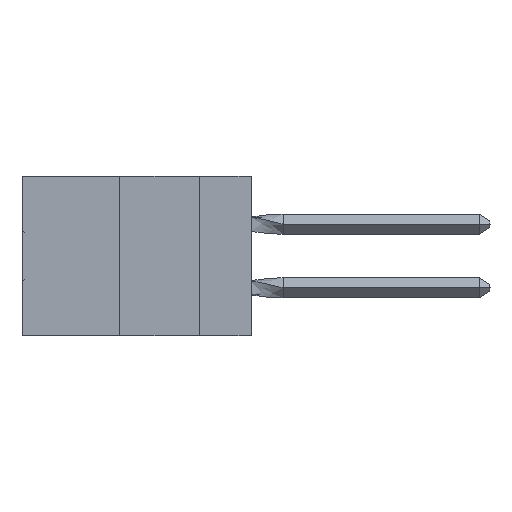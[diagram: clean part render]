
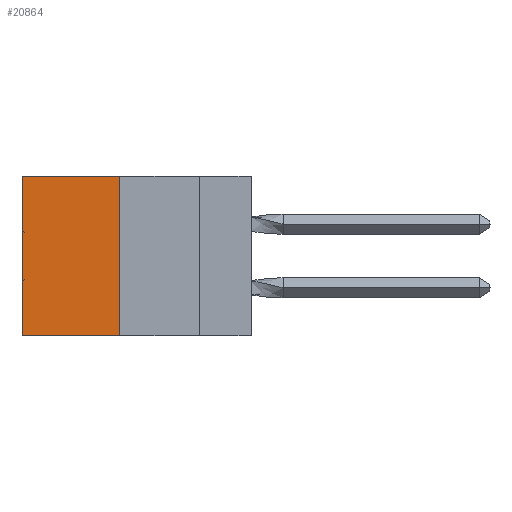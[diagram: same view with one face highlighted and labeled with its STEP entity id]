
A CAD part, left-side view. The second image highlights one B-rep face of the part: STEP entity #20864.
In plain terms, the highlighted planar face has unit normal (-1, 0, 0).
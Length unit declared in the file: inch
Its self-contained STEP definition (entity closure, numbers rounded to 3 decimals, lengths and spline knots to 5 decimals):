
#2740 = EDGE_CURVE ( 'NONE', #23271, #10534, #30842, .T. ) ;
#7665 = VECTOR ( 'NONE', #19204, 39.37008 ) ;
#10534 = VERTEX_POINT ( 'NONE', #34947 ) ;
#11364 = PLANE ( 'NONE',  #20987 ) ;
#13994 = EDGE_CURVE ( 'NONE', #23271, #24695, #32290, .T. ) ;
#16296 = LINE ( 'NONE', #21968, #38997 ) ;
#18318 = ORIENTED_EDGE ( 'NONE', *, *, #45078, .F. ) ;
#18521 = ORIENTED_EDGE ( 'NONE', *, *, #2740, .T. ) ;
#19204 = DIRECTION ( 'NONE',  ( 0., 1., 0. ) ) ;
#20609 = CARTESIAN_POINT ( 'NONE',  ( 0.305, 0.72, -0.5 ) ) ;
#20864 = ADVANCED_FACE ( 'NONE', ( #35247 ), #11364, .F. ) ;
#20987 = AXIS2_PLACEMENT_3D ( 'NONE', #46743, #35106, #39726 ) ;
#21790 = DIRECTION ( 'NONE',  ( 0., 0., -1. ) ) ;
#21948 = VECTOR ( 'NONE', #24195, 39.37008 ) ;
#21968 = CARTESIAN_POINT ( 'NONE',  ( 0.305, 0.72, -0.5 ) ) ;
#23271 = VERTEX_POINT ( 'NONE', #23732 ) ;
#23732 = CARTESIAN_POINT ( 'NONE',  ( 0.305, 0.413, 0. ) ) ;
#24195 = DIRECTION ( 'NONE',  ( 0., 0., -1. ) ) ;
#24695 = VERTEX_POINT ( 'NONE', #47883 ) ;
#30842 = LINE ( 'NONE', #46239, #7665 ) ;
#32054 = VECTOR ( 'NONE', #37929, 39.37008 ) ;
#32290 = LINE ( 'NONE', #43643, #21948 ) ;
#33954 = CARTESIAN_POINT ( 'NONE',  ( 0.305, 0.413, -0.5 ) ) ;
#34947 = CARTESIAN_POINT ( 'NONE',  ( 0.305, 0.72, 0. ) ) ;
#35106 = DIRECTION ( 'NONE',  ( 1., 0., 0. ) ) ;
#35247 = FACE_OUTER_BOUND ( 'NONE', #38164, .T. ) ;
#37929 = DIRECTION ( 'NONE',  ( 0., 1., 0. ) ) ;
#38164 = EDGE_LOOP ( 'NONE', ( #49173, #18318, #43894, #18521 ) ) ;
#38997 = VECTOR ( 'NONE', #21790, 39.37008 ) ;
#39726 = DIRECTION ( 'NONE',  ( 0., 0., -1. ) ) ;
#42832 = EDGE_CURVE ( 'NONE', #10534, #48463, #16296, .T. ) ;
#43643 = CARTESIAN_POINT ( 'NONE',  ( 0.305, 0.413, -0.5 ) ) ;
#43894 = ORIENTED_EDGE ( 'NONE', *, *, #13994, .F. ) ;
#45078 = EDGE_CURVE ( 'NONE', #24695, #48463, #48556, .T. ) ;
#46239 = CARTESIAN_POINT ( 'NONE',  ( 0.305, 0.413, 0. ) ) ;
#46743 = CARTESIAN_POINT ( 'NONE',  ( 0.305, 0.413, -0.5 ) ) ;
#47883 = CARTESIAN_POINT ( 'NONE',  ( 0.305, 0.413, -0.5 ) ) ;
#48463 = VERTEX_POINT ( 'NONE', #20609 ) ;
#48556 = LINE ( 'NONE', #33954, #32054 ) ;
#49173 = ORIENTED_EDGE ( 'NONE', *, *, #42832, .T. ) ;
